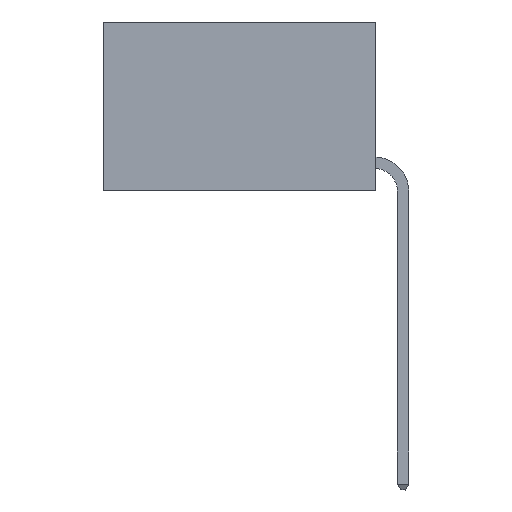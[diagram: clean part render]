
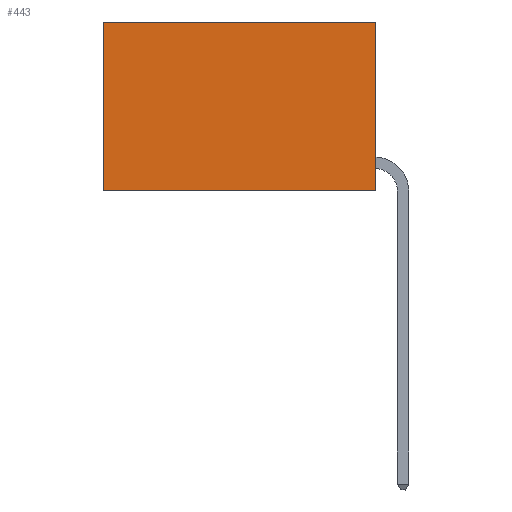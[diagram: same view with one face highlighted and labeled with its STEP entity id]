
A CAD part, left-side view. The second image highlights one B-rep face of the part: STEP entity #443.
In plain terms, the highlighted planar face has unit normal (-1, 0, 0).
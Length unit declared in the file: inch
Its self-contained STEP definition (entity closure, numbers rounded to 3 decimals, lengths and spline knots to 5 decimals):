
#44 = CARTESIAN_POINT ( 'NONE',  ( 0.2625, 0.6, -0.37 ) ) ;
#443 = ADVANCED_FACE ( 'NONE', ( #6482 ), #8240, .F. ) ;
#626 = VERTEX_POINT ( 'NONE', #5137 ) ;
#1079 = CARTESIAN_POINT ( 'NONE',  ( 0.2625, 0., 0. ) ) ;
#1816 = EDGE_CURVE ( 'NONE', #8649, #2926, #9047, .T. ) ;
#1890 = LINE ( 'NONE', #7877, #6354 ) ;
#2240 = VECTOR ( 'NONE', #3855, 39.37008 ) ;
#2435 = VECTOR ( 'NONE', #8969, 39.37008 ) ;
#2926 = VERTEX_POINT ( 'NONE', #44 ) ;
#3855 = DIRECTION ( 'NONE',  ( 0., 1., 0. ) ) ;
#4150 = DIRECTION ( 'NONE',  ( 0., 0., -1. ) ) ;
#4192 = CARTESIAN_POINT ( 'NONE',  ( 0.2625, 0., 0. ) ) ;
#4402 = VECTOR ( 'NONE', #10651, 39.37008 ) ;
#4629 = EDGE_CURVE ( 'NONE', #626, #10463, #9271, .T. ) ;
#4799 = LINE ( 'NONE', #7182, #2435 ) ;
#4924 = EDGE_LOOP ( 'NONE', ( #9380, #10557, #11222, #6690 ) ) ;
#5137 = CARTESIAN_POINT ( 'NONE',  ( 0.2625, 0., 0. ) ) ;
#5148 = CARTESIAN_POINT ( 'NONE',  ( 0.2625, 0.6, 0. ) ) ;
#6354 = VECTOR ( 'NONE', #8745, 39.37008 ) ;
#6482 = FACE_OUTER_BOUND ( 'NONE', #4924, .T. ) ;
#6631 = AXIS2_PLACEMENT_3D ( 'NONE', #4192, #8361, #4150 ) ;
#6690 = ORIENTED_EDGE ( 'NONE', *, *, #4629, .T. ) ;
#7182 = CARTESIAN_POINT ( 'NONE',  ( 0.2625, 0., 0. ) ) ;
#7877 = CARTESIAN_POINT ( 'NONE',  ( 0.2625, 0.6, 0. ) ) ;
#8240 = PLANE ( 'NONE',  #6631 ) ;
#8361 = DIRECTION ( 'NONE',  ( 1., 0., 0. ) ) ;
#8649 = VERTEX_POINT ( 'NONE', #8855 ) ;
#8745 = DIRECTION ( 'NONE',  ( 0., 0., -1. ) ) ;
#8855 = CARTESIAN_POINT ( 'NONE',  ( 0.2625, 0., -0.37 ) ) ;
#8969 = DIRECTION ( 'NONE',  ( 0., 0., -1. ) ) ;
#9047 = LINE ( 'NONE', #9816, #4402 ) ;
#9271 = LINE ( 'NONE', #1079, #2240 ) ;
#9380 = ORIENTED_EDGE ( 'NONE', *, *, #9437, .T. ) ;
#9437 = EDGE_CURVE ( 'NONE', #10463, #2926, #1890, .T. ) ;
#9816 = CARTESIAN_POINT ( 'NONE',  ( 0.2625, 0., -0.37 ) ) ;
#9997 = EDGE_CURVE ( 'NONE', #626, #8649, #4799, .T. ) ;
#10463 = VERTEX_POINT ( 'NONE', #5148 ) ;
#10557 = ORIENTED_EDGE ( 'NONE', *, *, #1816, .F. ) ;
#10651 = DIRECTION ( 'NONE',  ( 0., 1., 0. ) ) ;
#11222 = ORIENTED_EDGE ( 'NONE', *, *, #9997, .F. ) ;
